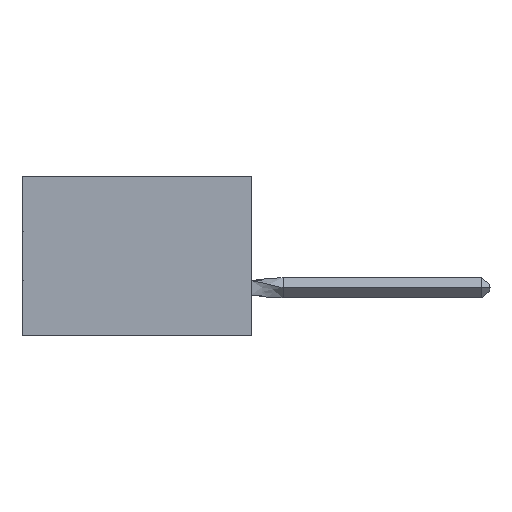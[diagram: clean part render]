
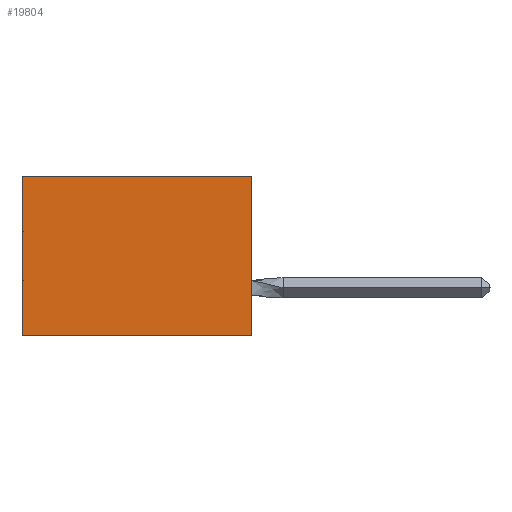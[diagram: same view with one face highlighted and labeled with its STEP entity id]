
A CAD part, left-side view. The second image highlights one B-rep face of the part: STEP entity #19804.
In plain terms, the highlighted planar face has unit normal (-1, 0, 0).
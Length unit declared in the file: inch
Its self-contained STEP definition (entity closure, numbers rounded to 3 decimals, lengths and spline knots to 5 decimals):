
#2056 = LINE ( 'NONE', #15540, #25675 ) ;
#3359 = VECTOR ( 'NONE', #10381, 39.37008 ) ;
#6618 = CARTESIAN_POINT ( 'NONE',  ( 0.305, 0., -0.5 ) ) ;
#7949 = DIRECTION ( 'NONE',  ( 0., 1., 0. ) ) ;
#8612 = LINE ( 'NONE', #46110, #30504 ) ;
#9828 = FACE_OUTER_BOUND ( 'NONE', #31968, .T. ) ;
#10381 = DIRECTION ( 'NONE',  ( 0., 1., 0. ) ) ;
#10817 = EDGE_CURVE ( 'NONE', #14094, #11319, #15745, .T. ) ;
#11319 = VERTEX_POINT ( 'NONE', #11878 ) ;
#11878 = CARTESIAN_POINT ( 'NONE',  ( 0.305, 0.72, -0.5 ) ) ;
#12301 = ORIENTED_EDGE ( 'NONE', *, *, #25853, .T. ) ;
#13298 = VECTOR ( 'NONE', #17988, 39.37008 ) ;
#14094 = VERTEX_POINT ( 'NONE', #20879 ) ;
#15540 = CARTESIAN_POINT ( 'NONE',  ( 0.305, 0., 0. ) ) ;
#15745 = LINE ( 'NONE', #6618, #3359 ) ;
#16248 = CARTESIAN_POINT ( 'NONE',  ( 0.305, 0., -0.5 ) ) ;
#17988 = DIRECTION ( 'NONE',  ( 0., 0., -1. ) ) ;
#18040 = VERTEX_POINT ( 'NONE', #35212 ) ;
#19804 = ADVANCED_FACE ( 'NONE', ( #9828 ), #35126, .F. ) ;
#20428 = DIRECTION ( 'NONE',  ( 1., 0., 0. ) ) ;
#20879 = CARTESIAN_POINT ( 'NONE',  ( 0.305, 0., -0.5 ) ) ;
#23399 = DIRECTION ( 'NONE',  ( 0., 0., -1. ) ) ;
#25675 = VECTOR ( 'NONE', #7949, 39.37008 ) ;
#25853 = EDGE_CURVE ( 'NONE', #35793, #18040, #2056, .T. ) ;
#28864 = AXIS2_PLACEMENT_3D ( 'NONE', #16248, #20428, #42573 ) ;
#30504 = VECTOR ( 'NONE', #23399, 39.37008 ) ;
#31968 = EDGE_LOOP ( 'NONE', ( #47134, #39103, #37120, #12301 ) ) ;
#34659 = LINE ( 'NONE', #40524, #13298 ) ;
#35126 = PLANE ( 'NONE',  #28864 ) ;
#35212 = CARTESIAN_POINT ( 'NONE',  ( 0.305, 0.72, 0. ) ) ;
#35793 = VERTEX_POINT ( 'NONE', #47208 ) ;
#37120 = ORIENTED_EDGE ( 'NONE', *, *, #42345, .F. ) ;
#39103 = ORIENTED_EDGE ( 'NONE', *, *, #10817, .F. ) ;
#40524 = CARTESIAN_POINT ( 'NONE',  ( 0.305, 0., -0.5 ) ) ;
#41342 = EDGE_CURVE ( 'NONE', #18040, #11319, #8612, .T. ) ;
#42345 = EDGE_CURVE ( 'NONE', #35793, #14094, #34659, .T. ) ;
#42573 = DIRECTION ( 'NONE',  ( 0., 0., -1. ) ) ;
#46110 = CARTESIAN_POINT ( 'NONE',  ( 0.305, 0.72, -0.5 ) ) ;
#47134 = ORIENTED_EDGE ( 'NONE', *, *, #41342, .T. ) ;
#47208 = CARTESIAN_POINT ( 'NONE',  ( 0.305, 0., 0. ) ) ;
